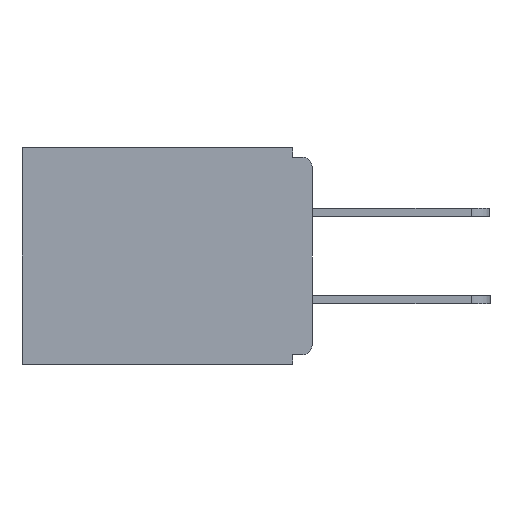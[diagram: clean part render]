
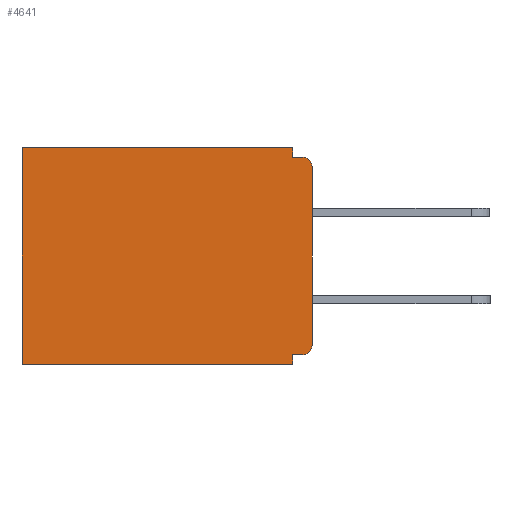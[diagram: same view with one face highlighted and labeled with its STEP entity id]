
A CAD part, left-side view. The second image highlights one B-rep face of the part: STEP entity #4641.
In plain terms, the highlighted planar face has unit normal (-1, 0, 0).
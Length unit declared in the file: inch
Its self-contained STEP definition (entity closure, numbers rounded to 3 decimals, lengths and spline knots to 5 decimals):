
#103 = VECTOR ( 'NONE', #4092, 39.37008 ) ;
#199 = CARTESIAN_POINT ( 'NONE',  ( 0.298, 0.015, -0.015 ) ) ;
#243 = CARTESIAN_POINT ( 'NONE',  ( 0.298, 0., -0.328 ) ) ;
#259 = DIRECTION ( 'NONE',  ( 0., 0., -1. ) ) ;
#452 = VERTEX_POINT ( 'NONE', #24309 ) ;
#851 = VECTOR ( 'NONE', #259, 39.37008 ) ;
#1402 = CARTESIAN_POINT ( 'NONE',  ( 0.298, 0.46, -0.343 ) ) ;
#1475 = EDGE_CURVE ( 'NONE', #16857, #14448, #23633, .T. ) ;
#1494 = DIRECTION ( 'NONE',  ( 0., 0., -1. ) ) ;
#3030 = LINE ( 'NONE', #23915, #28368 ) ;
#3251 = VECTOR ( 'NONE', #1494, 39.37008 ) ;
#4092 = DIRECTION ( 'NONE',  ( 0., 0., -1. ) ) ;
#4379 = DIRECTION ( 'NONE',  ( 0., 0., -1. ) ) ;
#4592 = LINE ( 'NONE', #13511, #103 ) ;
#4608 = ORIENTED_EDGE ( 'NONE', *, *, #6959, .T. ) ;
#4641 = ADVANCED_FACE ( 'NONE', ( #16438 ), #22393, .F. ) ;
#4809 = VERTEX_POINT ( 'NONE', #14606 ) ;
#5229 = EDGE_CURVE ( 'NONE', #16857, #18195, #16749, .T. ) ;
#6113 = VECTOR ( 'NONE', #17365, 39.37008 ) ;
#6565 = CARTESIAN_POINT ( 'NONE',  ( 0.298, 0., 0. ) ) ;
#6765 = DIRECTION ( 'NONE',  ( 0., 0., -1. ) ) ;
#6959 = EDGE_CURVE ( 'NONE', #4809, #14058, #26754, .T. ) ;
#7678 = EDGE_CURVE ( 'NONE', #29404, #14058, #28881, .T. ) ;
#7810 = CARTESIAN_POINT ( 'NONE',  ( 0.298, 0.015, -0.328 ) ) ;
#8106 = VECTOR ( 'NONE', #18684, 39.37008 ) ;
#8381 = CARTESIAN_POINT ( 'NONE',  ( 0.298, 0.015, -0.03 ) ) ;
#8579 = CARTESIAN_POINT ( 'NONE',  ( 0.298, 0.46, 0. ) ) ;
#8770 = EDGE_LOOP ( 'NONE', ( #12898, #19862, #16414, #25937, #4608, #20423, #26864, #29069, #25819, #29780 ) ) ;
#9707 = VERTEX_POINT ( 'NONE', #21085 ) ;
#9766 = CARTESIAN_POINT ( 'NONE',  ( 0.298, 0., -0.313 ) ) ;
#10748 = CARTESIAN_POINT ( 'NONE',  ( 0.298, 0., 0. ) ) ;
#11109 = CARTESIAN_POINT ( 'NONE',  ( 0.298, 0., -0.015 ) ) ;
#11925 = AXIS2_PLACEMENT_3D ( 'NONE', #13907, #30469, #4379 ) ;
#12069 = DIRECTION ( 'NONE',  ( 0., 1., 0. ) ) ;
#12812 = CIRCLE ( 'NONE', #11925, 0.015 ) ;
#12898 = ORIENTED_EDGE ( 'NONE', *, *, #5229, .T. ) ;
#13292 = CARTESIAN_POINT ( 'NONE',  ( 0.298, 0.031, -0.343 ) ) ;
#13511 = CARTESIAN_POINT ( 'NONE',  ( 0.298, 0.031, -0.343 ) ) ;
#13907 = CARTESIAN_POINT ( 'NONE',  ( 0.298, 0.015, -0.313 ) ) ;
#14058 = VERTEX_POINT ( 'NONE', #1402 ) ;
#14067 = EDGE_CURVE ( 'NONE', #452, #18195, #27890, .T. ) ;
#14448 = VERTEX_POINT ( 'NONE', #9766 ) ;
#14606 = CARTESIAN_POINT ( 'NONE',  ( 0.298, 0.46, 0. ) ) ;
#14859 = CARTESIAN_POINT ( 'NONE',  ( 0.298, 0.031, -0.328 ) ) ;
#15003 = AXIS2_PLACEMENT_3D ( 'NONE', #8381, #15294, #27202 ) ;
#15294 = DIRECTION ( 'NONE',  ( -1., 0., 0. ) ) ;
#15800 = EDGE_CURVE ( 'NONE', #9707, #452, #21538, .T. ) ;
#16046 = DIRECTION ( 'NONE',  ( 0., -1., 0. ) ) ;
#16312 = CARTESIAN_POINT ( 'NONE',  ( 0.298, 0., -0.343 ) ) ;
#16414 = ORIENTED_EDGE ( 'NONE', *, *, #15800, .F. ) ;
#16438 = FACE_OUTER_BOUND ( 'NONE', #8770, .T. ) ;
#16749 = CIRCLE ( 'NONE', #15003, 0.015 ) ;
#16857 = VERTEX_POINT ( 'NONE', #25749 ) ;
#17365 = DIRECTION ( 'NONE',  ( 0., 1., 0. ) ) ;
#17739 = EDGE_CURVE ( 'NONE', #27409, #25178, #25857, .T. ) ;
#17863 = EDGE_CURVE ( 'NONE', #25178, #29404, #4592, .T. ) ;
#18195 = VERTEX_POINT ( 'NONE', #199 ) ;
#18684 = DIRECTION ( 'NONE',  ( 0., 1., 0. ) ) ;
#19862 = ORIENTED_EDGE ( 'NONE', *, *, #14067, .F. ) ;
#20423 = ORIENTED_EDGE ( 'NONE', *, *, #7678, .F. ) ;
#20807 = EDGE_CURVE ( 'NONE', #27409, #14448, #12812, .T. ) ;
#21085 = CARTESIAN_POINT ( 'NONE',  ( 0.298, 0.031, 0. ) ) ;
#21538 = LINE ( 'NONE', #13292, #24872 ) ;
#21568 = AXIS2_PLACEMENT_3D ( 'NONE', #6565, #27967, #6765 ) ;
#22342 = VECTOR ( 'NONE', #16046, 39.37008 ) ;
#22393 = PLANE ( 'NONE',  #21568 ) ;
#23214 = CARTESIAN_POINT ( 'NONE',  ( 0.298, 0.031, -0.343 ) ) ;
#23633 = LINE ( 'NONE', #10748, #851 ) ;
#23915 = CARTESIAN_POINT ( 'NONE',  ( 0.298, 0., 0. ) ) ;
#24309 = CARTESIAN_POINT ( 'NONE',  ( 0.298, 0.031, -0.015 ) ) ;
#24872 = VECTOR ( 'NONE', #30150, 39.37008 ) ;
#25178 = VERTEX_POINT ( 'NONE', #14859 ) ;
#25749 = CARTESIAN_POINT ( 'NONE',  ( 0.298, 0., -0.03 ) ) ;
#25819 = ORIENTED_EDGE ( 'NONE', *, *, #20807, .T. ) ;
#25857 = LINE ( 'NONE', #243, #6113 ) ;
#25937 = ORIENTED_EDGE ( 'NONE', *, *, #27686, .T. ) ;
#26754 = LINE ( 'NONE', #8579, #3251 ) ;
#26864 = ORIENTED_EDGE ( 'NONE', *, *, #17863, .F. ) ;
#27202 = DIRECTION ( 'NONE',  ( 0., 0., -1. ) ) ;
#27409 = VERTEX_POINT ( 'NONE', #7810 ) ;
#27686 = EDGE_CURVE ( 'NONE', #9707, #4809, #3030, .T. ) ;
#27890 = LINE ( 'NONE', #11109, #22342 ) ;
#27967 = DIRECTION ( 'NONE',  ( 1., 0., 0. ) ) ;
#28368 = VECTOR ( 'NONE', #12069, 39.37008 ) ;
#28881 = LINE ( 'NONE', #16312, #8106 ) ;
#29069 = ORIENTED_EDGE ( 'NONE', *, *, #17739, .F. ) ;
#29404 = VERTEX_POINT ( 'NONE', #23214 ) ;
#29780 = ORIENTED_EDGE ( 'NONE', *, *, #1475, .F. ) ;
#30150 = DIRECTION ( 'NONE',  ( 0., 0., -1. ) ) ;
#30469 = DIRECTION ( 'NONE',  ( -1., 0., 0. ) ) ;
